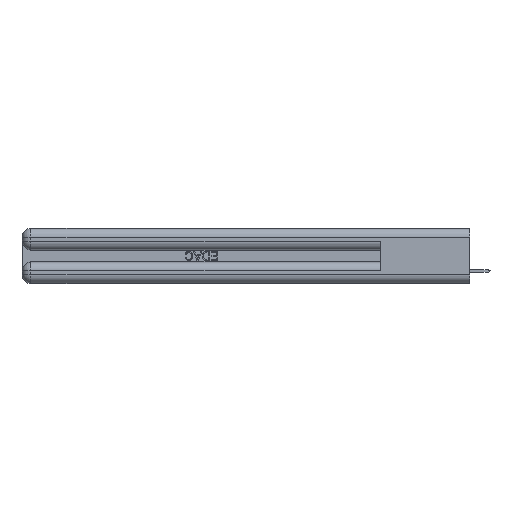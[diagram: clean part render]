
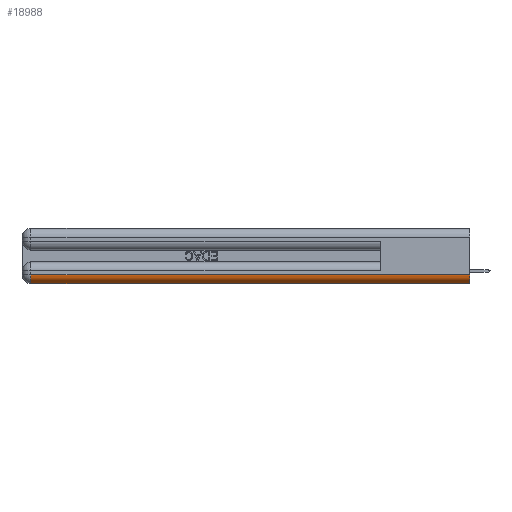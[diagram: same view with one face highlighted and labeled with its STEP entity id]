
A CAD part, left-side view. The second image highlights one B-rep face of the part: STEP entity #18988.
In plain terms, the highlighted cylindrical face has radius 1.524 mm (diameter 3.048 mm), a partial arc.
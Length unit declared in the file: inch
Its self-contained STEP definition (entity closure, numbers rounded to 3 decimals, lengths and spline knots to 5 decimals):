
#200 = EDGE_CURVE ( 'NONE', #36735, #30146, #27303, .T. ) ;
#1748 = ORIENTED_EDGE ( 'NONE', *, *, #46154, .F. ) ;
#3566 = DIRECTION ( 'NONE',  ( 0., -1., 0. ) ) ;
#3837 = CARTESIAN_POINT ( 'NONE',  ( 0.06, 0., 0.06 ) ) ;
#7764 = VECTOR ( 'NONE', #48694, 39.37008 ) ;
#8564 = CARTESIAN_POINT ( 'NONE',  ( 0., 0., 0.06 ) ) ;
#10096 = EDGE_LOOP ( 'NONE', ( #49258, #1748, #29147, #15209 ) ) ;
#12907 = CIRCLE ( 'NONE', #31978, 0.06 ) ;
#13891 = LINE ( 'NONE', #8564, #50226 ) ;
#13928 = CARTESIAN_POINT ( 'NONE',  ( 0.06, 0., 0. ) ) ;
#15209 = ORIENTED_EDGE ( 'NONE', *, *, #200, .F. ) ;
#16518 = FACE_OUTER_BOUND ( 'NONE', #10096, .T. ) ;
#17175 = VERTEX_POINT ( 'NONE', #50186 ) ;
#18969 = AXIS2_PLACEMENT_3D ( 'NONE', #23057, #52040, #22506 ) ;
#18988 = ADVANCED_FACE ( 'NONE', ( #16518 ), #33080, .T. ) ;
#21026 = DIRECTION ( 'NONE',  ( 0., -1., 0. ) ) ;
#21119 = DIRECTION ( 'NONE',  ( 0., 1., 0. ) ) ;
#21274 = AXIS2_PLACEMENT_3D ( 'NONE', #49870, #21119, #41991 ) ;
#21447 = CARTESIAN_POINT ( 'NONE',  ( 0., 0., 0.06 ) ) ;
#22506 = DIRECTION ( 'NONE',  ( 0., 0., 1. ) ) ;
#23057 = CARTESIAN_POINT ( 'NONE',  ( 0.06, 2.94, 0.06 ) ) ;
#24955 = VERTEX_POINT ( 'NONE', #21447 ) ;
#27303 = LINE ( 'NONE', #35713, #7764 ) ;
#29147 = ORIENTED_EDGE ( 'NONE', *, *, #45362, .F. ) ;
#30146 = VERTEX_POINT ( 'NONE', #47583 ) ;
#31978 = AXIS2_PLACEMENT_3D ( 'NONE', #3837, #3566, #48840 ) ;
#33080 = CYLINDRICAL_SURFACE ( 'NONE', #21274, 0.06 ) ;
#35713 = CARTESIAN_POINT ( 'NONE',  ( 0.06, 3., 0. ) ) ;
#36735 = VERTEX_POINT ( 'NONE', #13928 ) ;
#41991 = DIRECTION ( 'NONE',  ( 0., 0., 1. ) ) ;
#45113 = EDGE_CURVE ( 'NONE', #24955, #36735, #12907, .T. ) ;
#45362 = EDGE_CURVE ( 'NONE', #30146, #17175, #50110, .T. ) ;
#46154 = EDGE_CURVE ( 'NONE', #17175, #24955, #13891, .T. ) ;
#47583 = CARTESIAN_POINT ( 'NONE',  ( 0.06, 2.94, 0. ) ) ;
#48694 = DIRECTION ( 'NONE',  ( 0., 1., 0. ) ) ;
#48840 = DIRECTION ( 'NONE',  ( 0., 0., 1. ) ) ;
#49258 = ORIENTED_EDGE ( 'NONE', *, *, #45113, .F. ) ;
#49870 = CARTESIAN_POINT ( 'NONE',  ( 0.06, 0., 0.06 ) ) ;
#50110 = CIRCLE ( 'NONE', #18969, 0.06 ) ;
#50186 = CARTESIAN_POINT ( 'NONE',  ( 0., 2.94, 0.06 ) ) ;
#50226 = VECTOR ( 'NONE', #21026, 39.37008 ) ;
#52040 = DIRECTION ( 'NONE',  ( 0., 1., 0. ) ) ;
